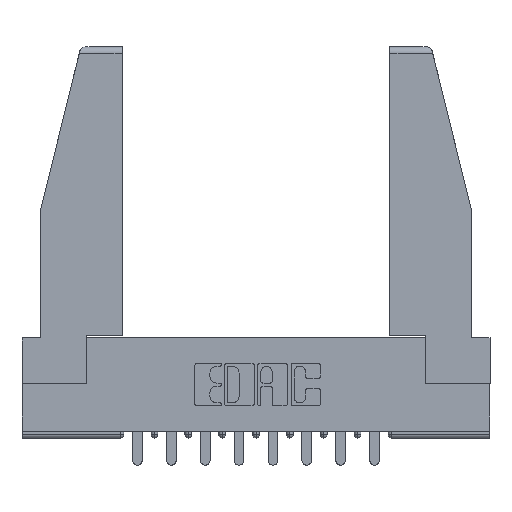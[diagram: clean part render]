
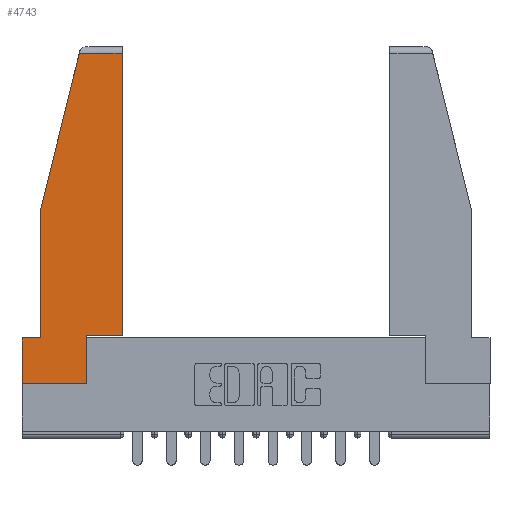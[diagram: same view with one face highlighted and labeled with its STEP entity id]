
A CAD part, top view. The second image highlights one B-rep face of the part: STEP entity #4743.
In plain terms, the highlighted planar face has unit normal (0, 0, 1).
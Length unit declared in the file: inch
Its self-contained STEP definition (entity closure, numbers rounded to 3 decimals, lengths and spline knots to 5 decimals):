
#458 = DIRECTION ( 'NONE',  ( 1., 0., 0. ) ) ;
#759 = LINE ( 'NONE', #2813, #2046 ) ;
#929 = LINE ( 'NONE', #9525, #6242 ) ;
#1028 = ORIENTED_EDGE ( 'NONE', *, *, #4695, .T. ) ;
#1239 = VERTEX_POINT ( 'NONE', #10813 ) ;
#1382 = VERTEX_POINT ( 'NONE', #3028 ) ;
#1574 = ORIENTED_EDGE ( 'NONE', *, *, #6571, .T. ) ;
#1794 = LINE ( 'NONE', #4689, #11132 ) ;
#1843 = VECTOR ( 'NONE', #7110, 39.37008 ) ;
#2046 = VECTOR ( 'NONE', #14254, 39.37008 ) ;
#2141 = VERTEX_POINT ( 'NONE', #14144 ) ;
#2813 = CARTESIAN_POINT ( 'NONE',  ( 0.271, 1.55, 0. ) ) ;
#3028 = CARTESIAN_POINT ( 'NONE',  ( 0.461, 1.52, 0. ) ) ;
#3576 = DIRECTION ( 'NONE',  ( 1., 0., 0. ) ) ;
#3908 = VECTOR ( 'NONE', #9503, 39.37008 ) ;
#3978 = ORIENTED_EDGE ( 'NONE', *, *, #8844, .T. ) ;
#4089 = ORIENTED_EDGE ( 'NONE', *, *, #4824, .T. ) ;
#4118 = ORIENTED_EDGE ( 'NONE', *, *, #12571, .T. ) ;
#4212 = VECTOR ( 'NONE', #6229, 39.37008 ) ;
#4227 = CARTESIAN_POINT ( 'NONE',  ( 0.297, 0., 0. ) ) ;
#4689 = CARTESIAN_POINT ( 'NONE',  ( 0., 0.21, 0. ) ) ;
#4695 = EDGE_CURVE ( 'NONE', #11719, #13346, #9173, .T. ) ;
#4743 = ADVANCED_FACE ( 'NONE', ( #9932 ), #6278, .T. ) ;
#4824 = EDGE_CURVE ( 'NONE', #2141, #7872, #9533, .T. ) ;
#5007 = CARTESIAN_POINT ( 'NONE',  ( 0., 0., 0. ) ) ;
#5453 = EDGE_LOOP ( 'NONE', ( #7423, #5506, #8639, #4089, #3978, #1574, #4118, #5543, #1028 ) ) ;
#5506 = ORIENTED_EDGE ( 'NONE', *, *, #8210, .T. ) ;
#5543 = ORIENTED_EDGE ( 'NONE', *, *, #13820, .T. ) ;
#5556 = LINE ( 'NONE', #5945, #3908 ) ;
#5945 = CARTESIAN_POINT ( 'NONE',  ( 0.461, 0.223, 0. ) ) ;
#6098 = LINE ( 'NONE', #6840, #8864 ) ;
#6229 = DIRECTION ( 'NONE',  ( 0., -1., 0. ) ) ;
#6242 = VECTOR ( 'NONE', #3576, 39.37008 ) ;
#6278 = PLANE ( 'NONE',  #13664 ) ;
#6571 = EDGE_CURVE ( 'NONE', #10763, #10108, #1794, .T. ) ;
#6840 = CARTESIAN_POINT ( 'NONE',  ( 0., 1.52, 0. ) ) ;
#7110 = DIRECTION ( 'NONE',  ( 1., 0., 0. ) ) ;
#7399 = DIRECTION ( 'NONE',  ( 0., -1., 0. ) ) ;
#7423 = ORIENTED_EDGE ( 'NONE', *, *, #10644, .T. ) ;
#7464 = DIRECTION ( 'NONE',  ( 0., 0., 1. ) ) ;
#7872 = VERTEX_POINT ( 'NONE', #10705 ) ;
#8021 = DIRECTION ( 'NONE',  ( -1., 0., 0. ) ) ;
#8210 = EDGE_CURVE ( 'NONE', #1382, #14638, #6098, .T. ) ;
#8639 = ORIENTED_EDGE ( 'NONE', *, *, #12675, .T. ) ;
#8844 = EDGE_CURVE ( 'NONE', #7872, #10763, #12170, .T. ) ;
#8864 = VECTOR ( 'NONE', #8021, 39.37008 ) ;
#9173 = LINE ( 'NONE', #11728, #1843 ) ;
#9503 = DIRECTION ( 'NONE',  ( 0., 1., 0. ) ) ;
#9512 = VECTOR ( 'NONE', #12422, 39.37008 ) ;
#9525 = CARTESIAN_POINT ( 'NONE',  ( 0., 0., 0. ) ) ;
#9533 = LINE ( 'NONE', #11007, #4212 ) ;
#9932 = FACE_OUTER_BOUND ( 'NONE', #5453, .T. ) ;
#10108 = VERTEX_POINT ( 'NONE', #11536 ) ;
#10511 = DIRECTION ( 'NONE',  ( -1., 0., 0. ) ) ;
#10572 = LINE ( 'NONE', #4227, #9512 ) ;
#10644 = EDGE_CURVE ( 'NONE', #13346, #1382, #5556, .T. ) ;
#10705 = CARTESIAN_POINT ( 'NONE',  ( 0.086, 0.21, 0. ) ) ;
#10763 = VERTEX_POINT ( 'NONE', #14182 ) ;
#10813 = CARTESIAN_POINT ( 'NONE',  ( 0.297, 0., 0. ) ) ;
#11007 = CARTESIAN_POINT ( 'NONE',  ( 0.086, 0.8, 0. ) ) ;
#11132 = VECTOR ( 'NONE', #7399, 39.37008 ) ;
#11251 = VECTOR ( 'NONE', #10511, 39.37008 ) ;
#11536 = CARTESIAN_POINT ( 'NONE',  ( 0., 0., 0. ) ) ;
#11719 = VERTEX_POINT ( 'NONE', #13643 ) ;
#11728 = CARTESIAN_POINT ( 'NONE',  ( 0.297, 0.223, 0. ) ) ;
#11987 = CARTESIAN_POINT ( 'NONE',  ( 0.2636, 1.52, 0. ) ) ;
#12170 = LINE ( 'NONE', #13804, #11251 ) ;
#12422 = DIRECTION ( 'NONE',  ( 0., 1., 0. ) ) ;
#12571 = EDGE_CURVE ( 'NONE', #10108, #1239, #929, .T. ) ;
#12675 = EDGE_CURVE ( 'NONE', #14638, #2141, #759, .T. ) ;
#13244 = CARTESIAN_POINT ( 'NONE',  ( 0.461, 0.223, 0. ) ) ;
#13346 = VERTEX_POINT ( 'NONE', #13244 ) ;
#13643 = CARTESIAN_POINT ( 'NONE',  ( 0.297, 0.223, 0. ) ) ;
#13664 = AXIS2_PLACEMENT_3D ( 'NONE', #5007, #7464, #458 ) ;
#13804 = CARTESIAN_POINT ( 'NONE',  ( 0., 0.21, 0. ) ) ;
#13820 = EDGE_CURVE ( 'NONE', #1239, #11719, #10572, .T. ) ;
#14144 = CARTESIAN_POINT ( 'NONE',  ( 0.086, 0.8, 0. ) ) ;
#14182 = CARTESIAN_POINT ( 'NONE',  ( 0., 0.21, 0. ) ) ;
#14254 = DIRECTION ( 'NONE',  ( -0.239, -0.971, 0. ) ) ;
#14638 = VERTEX_POINT ( 'NONE', #11987 ) ;
